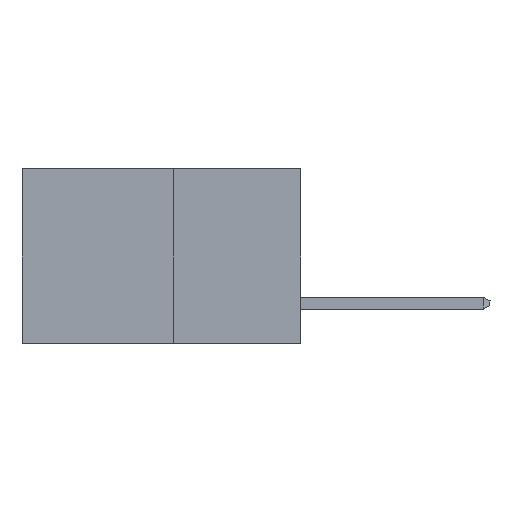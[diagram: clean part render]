
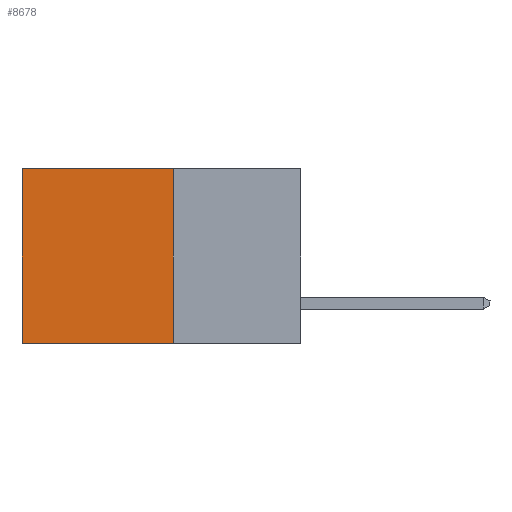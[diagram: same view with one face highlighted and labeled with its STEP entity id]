
A CAD part, left-side view. The second image highlights one B-rep face of the part: STEP entity #8678.
In plain terms, the highlighted planar face has unit normal (-1, 0, 0).
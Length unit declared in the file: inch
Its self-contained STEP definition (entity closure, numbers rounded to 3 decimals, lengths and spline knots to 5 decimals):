
#3624 = VERTEX_POINT ( 'NONE', #19549 ) ;
#6812 = CARTESIAN_POINT ( 'NONE',  ( 0.277, 0.59, 0. ) ) ;
#6853 = ORIENTED_EDGE ( 'NONE', *, *, #13880, .F. ) ;
#7437 = CARTESIAN_POINT ( 'NONE',  ( 0.277, 0.27, -0.37 ) ) ;
#7648 = VECTOR ( 'NONE', #12293, 39.37008 ) ;
#8678 = ADVANCED_FACE ( 'NONE', ( #12668 ), #15629, .F. ) ;
#9527 = DIRECTION ( 'NONE',  ( 1., 0., 0. ) ) ;
#9529 = CARTESIAN_POINT ( 'NONE',  ( 0.277, 0.27, 0. ) ) ;
#9724 = EDGE_CURVE ( 'NONE', #14389, #3624, #19006, .T. ) ;
#10026 = LINE ( 'NONE', #10146, #20950 ) ;
#10096 = ORIENTED_EDGE ( 'NONE', *, *, #9724, .T. ) ;
#10146 = CARTESIAN_POINT ( 'NONE',  ( 0.277, 0.27, -0.37 ) ) ;
#11600 = LINE ( 'NONE', #22088, #26668 ) ;
#12293 = DIRECTION ( 'NONE',  ( 0., 1., 0. ) ) ;
#12668 = FACE_OUTER_BOUND ( 'NONE', #20369, .T. ) ;
#13665 = ORIENTED_EDGE ( 'NONE', *, *, #18713, .T. ) ;
#13880 = EDGE_CURVE ( 'NONE', #23268, #22030, #10026, .T. ) ;
#14364 = CARTESIAN_POINT ( 'NONE',  ( 0.277, 0.27, 0. ) ) ;
#14389 = VERTEX_POINT ( 'NONE', #6812 ) ;
#15629 = PLANE ( 'NONE',  #21478 ) ;
#17337 = EDGE_CURVE ( 'NONE', #22030, #3624, #11600, .T. ) ;
#17977 = DIRECTION ( 'NONE',  ( 0., 1., 0. ) ) ;
#18713 = EDGE_CURVE ( 'NONE', #23268, #14389, #24086, .T. ) ;
#19006 = LINE ( 'NONE', #20984, #24519 ) ;
#19549 = CARTESIAN_POINT ( 'NONE',  ( 0.277, 0.59, -0.37 ) ) ;
#20062 = ORIENTED_EDGE ( 'NONE', *, *, #17337, .F. ) ;
#20369 = EDGE_LOOP ( 'NONE', ( #10096, #20062, #6853, #13665 ) ) ;
#20950 = VECTOR ( 'NONE', #22502, 39.37008 ) ;
#20984 = CARTESIAN_POINT ( 'NONE',  ( 0.277, 0.59, -0.37 ) ) ;
#21478 = AXIS2_PLACEMENT_3D ( 'NONE', #7437, #9527, #23930 ) ;
#22030 = VERTEX_POINT ( 'NONE', #24979 ) ;
#22088 = CARTESIAN_POINT ( 'NONE',  ( 0.277, 0.27, -0.37 ) ) ;
#22502 = DIRECTION ( 'NONE',  ( 0., 0., -1. ) ) ;
#23083 = DIRECTION ( 'NONE',  ( 0., 0., -1. ) ) ;
#23268 = VERTEX_POINT ( 'NONE', #9529 ) ;
#23930 = DIRECTION ( 'NONE',  ( 0., 0., -1. ) ) ;
#24086 = LINE ( 'NONE', #14364, #7648 ) ;
#24519 = VECTOR ( 'NONE', #23083, 39.37008 ) ;
#24979 = CARTESIAN_POINT ( 'NONE',  ( 0.277, 0.27, -0.37 ) ) ;
#26668 = VECTOR ( 'NONE', #17977, 39.37008 ) ;
